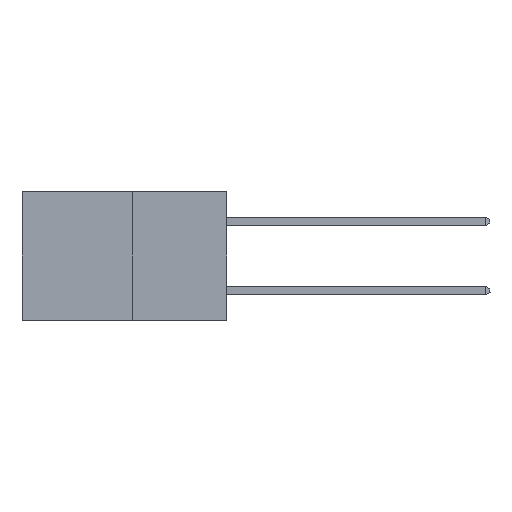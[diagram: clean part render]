
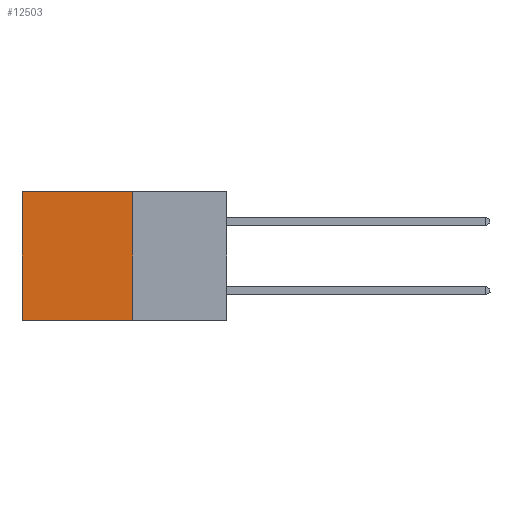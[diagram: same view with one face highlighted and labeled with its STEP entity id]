
A CAD part, left-side view. The second image highlights one B-rep face of the part: STEP entity #12503.
In plain terms, the highlighted planar face has unit normal (-1, 0, 0).
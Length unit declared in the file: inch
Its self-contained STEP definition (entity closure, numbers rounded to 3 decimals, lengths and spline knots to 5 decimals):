
#5 = CARTESIAN_POINT ( 'NONE',  ( 0.277, 0.59, 0. ) ) ;
#1171 = LINE ( 'NONE', #10754, #9908 ) ;
#1850 = CARTESIAN_POINT ( 'NONE',  ( 0.277, 0.27, -0.37 ) ) ;
#1920 = ORIENTED_EDGE ( 'NONE', *, *, #4273, .T. ) ;
#2205 = EDGE_CURVE ( 'NONE', #13993, #4585, #1171, .T. ) ;
#2578 = DIRECTION ( 'NONE',  ( 0., 0., -1. ) ) ;
#2943 = VECTOR ( 'NONE', #2578, 39.37008 ) ;
#3198 = CARTESIAN_POINT ( 'NONE',  ( 0.277, 0.59, -0.37 ) ) ;
#3200 = LINE ( 'NONE', #3896, #5882 ) ;
#3736 = ORIENTED_EDGE ( 'NONE', *, *, #2205, .T. ) ;
#3753 = PLANE ( 'NONE',  #12148 ) ;
#3799 = CARTESIAN_POINT ( 'NONE',  ( 0.277, 0.27, -0.37 ) ) ;
#3896 = CARTESIAN_POINT ( 'NONE',  ( 0.277, 0.59, -0.37 ) ) ;
#4273 = EDGE_CURVE ( 'NONE', #4585, #8204, #3200, .T. ) ;
#4320 = EDGE_CURVE ( 'NONE', #4549, #8204, #8582, .T. ) ;
#4549 = VERTEX_POINT ( 'NONE', #9198 ) ;
#4585 = VERTEX_POINT ( 'NONE', #5 ) ;
#4939 = DIRECTION ( 'NONE',  ( 1., 0., 0. ) ) ;
#4959 = ORIENTED_EDGE ( 'NONE', *, *, #4320, .F. ) ;
#5882 = VECTOR ( 'NONE', #11937, 39.37008 ) ;
#6058 = ORIENTED_EDGE ( 'NONE', *, *, #6719, .F. ) ;
#6719 = EDGE_CURVE ( 'NONE', #13993, #4549, #9363, .T. ) ;
#8204 = VERTEX_POINT ( 'NONE', #3198 ) ;
#8380 = DIRECTION ( 'NONE',  ( 0., 1., 0. ) ) ;
#8582 = LINE ( 'NONE', #1850, #11113 ) ;
#9198 = CARTESIAN_POINT ( 'NONE',  ( 0.277, 0.27, -0.37 ) ) ;
#9363 = LINE ( 'NONE', #9395, #2943 ) ;
#9395 = CARTESIAN_POINT ( 'NONE',  ( 0.277, 0.27, -0.37 ) ) ;
#9699 = EDGE_LOOP ( 'NONE', ( #1920, #4959, #6058, #3736 ) ) ;
#9908 = VECTOR ( 'NONE', #10114, 39.37008 ) ;
#10114 = DIRECTION ( 'NONE',  ( 0., 1., 0. ) ) ;
#10754 = CARTESIAN_POINT ( 'NONE',  ( 0.277, 0.27, 0. ) ) ;
#11113 = VECTOR ( 'NONE', #8380, 39.37008 ) ;
#11937 = DIRECTION ( 'NONE',  ( 0., 0., -1. ) ) ;
#12079 = CARTESIAN_POINT ( 'NONE',  ( 0.277, 0.27, 0. ) ) ;
#12148 = AXIS2_PLACEMENT_3D ( 'NONE', #3799, #4939, #12769 ) ;
#12503 = ADVANCED_FACE ( 'NONE', ( #13244 ), #3753, .F. ) ;
#12769 = DIRECTION ( 'NONE',  ( 0., 0., -1. ) ) ;
#13244 = FACE_OUTER_BOUND ( 'NONE', #9699, .T. ) ;
#13993 = VERTEX_POINT ( 'NONE', #12079 ) ;
